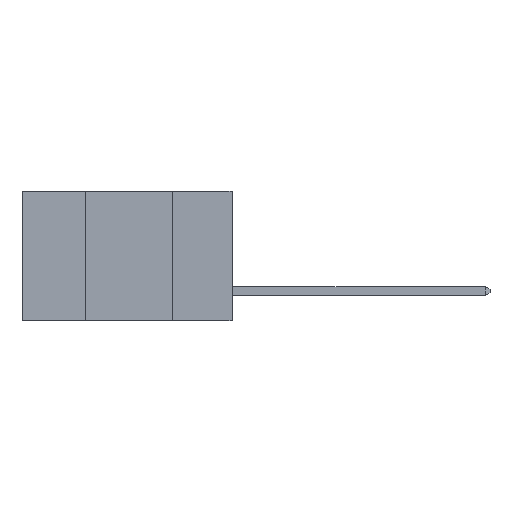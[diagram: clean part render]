
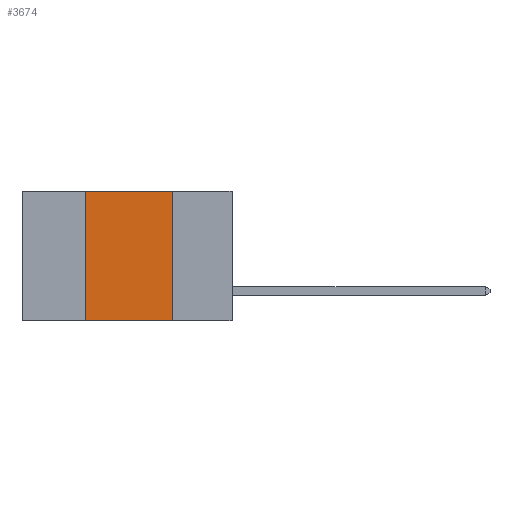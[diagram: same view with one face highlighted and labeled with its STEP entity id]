
A CAD part, left-side view. The second image highlights one B-rep face of the part: STEP entity #3674.
In plain terms, the highlighted planar face has unit normal (-1, 0, 0).
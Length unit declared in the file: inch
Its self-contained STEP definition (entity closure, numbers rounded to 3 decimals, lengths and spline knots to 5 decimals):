
#376 = DIRECTION ( 'NONE',  ( 0., -1., 0. ) ) ;
#1251 = EDGE_CURVE ( 'NONE', #8617, #5970, #23182, .T. ) ;
#1689 = CARTESIAN_POINT ( 'NONE',  ( 0., 0.17, -0.37 ) ) ;
#1973 = CARTESIAN_POINT ( 'NONE',  ( 0., 0.17, 0. ) ) ;
#3674 = ADVANCED_FACE ( 'NONE', ( #11266 ), #14317, .F. ) ;
#4388 = VERTEX_POINT ( 'NONE', #1689 ) ;
#5970 = VERTEX_POINT ( 'NONE', #6636 ) ;
#6085 = EDGE_CURVE ( 'NONE', #9747, #8617, #6362, .T. ) ;
#6362 = LINE ( 'NONE', #8987, #15832 ) ;
#6636 = CARTESIAN_POINT ( 'NONE',  ( 0., 0.17, 0. ) ) ;
#7655 = AXIS2_PLACEMENT_3D ( 'NONE', #13790, #13759, #13734 ) ;
#8255 = CARTESIAN_POINT ( 'NONE',  ( 0., 0.42, 0. ) ) ;
#8513 = VECTOR ( 'NONE', #15429, 39.37008 ) ;
#8617 = VERTEX_POINT ( 'NONE', #8255 ) ;
#8987 = CARTESIAN_POINT ( 'NONE',  ( 0., 0.42, 0. ) ) ;
#9747 = VERTEX_POINT ( 'NONE', #13325 ) ;
#10150 = ORIENTED_EDGE ( 'NONE', *, *, #6085, .F. ) ;
#10874 = DIRECTION ( 'NONE',  ( 0., 0., 1. ) ) ;
#11072 = EDGE_CURVE ( 'NONE', #5970, #4388, #22923, .T. ) ;
#11266 = FACE_OUTER_BOUND ( 'NONE', #13782, .T. ) ;
#11583 = DIRECTION ( 'NONE',  ( 0., -1., 0. ) ) ;
#11943 = CARTESIAN_POINT ( 'NONE',  ( 0., 0.6, 0. ) ) ;
#13325 = CARTESIAN_POINT ( 'NONE',  ( 0., 0.42, -0.37 ) ) ;
#13734 = DIRECTION ( 'NONE',  ( 0., 0., -1. ) ) ;
#13759 = DIRECTION ( 'NONE',  ( 1., 0., 0. ) ) ;
#13782 = EDGE_LOOP ( 'NONE', ( #18398, #23372, #10150, #17527 ) ) ;
#13790 = CARTESIAN_POINT ( 'NONE',  ( 0., 0.6, 0. ) ) ;
#14317 = PLANE ( 'NONE',  #7655 ) ;
#14659 = LINE ( 'NONE', #17742, #24613 ) ;
#15429 = DIRECTION ( 'NONE',  ( 0., 0., -1. ) ) ;
#15832 = VECTOR ( 'NONE', #10874, 39.37008 ) ;
#17527 = ORIENTED_EDGE ( 'NONE', *, *, #19955, .T. ) ;
#17742 = CARTESIAN_POINT ( 'NONE',  ( 0., 0.6, -0.37 ) ) ;
#18210 = VECTOR ( 'NONE', #11583, 39.37008 ) ;
#18398 = ORIENTED_EDGE ( 'NONE', *, *, #11072, .F. ) ;
#19955 = EDGE_CURVE ( 'NONE', #9747, #4388, #14659, .T. ) ;
#22923 = LINE ( 'NONE', #1973, #8513 ) ;
#23182 = LINE ( 'NONE', #11943, #18210 ) ;
#23372 = ORIENTED_EDGE ( 'NONE', *, *, #1251, .F. ) ;
#24613 = VECTOR ( 'NONE', #376, 39.37008 ) ;
